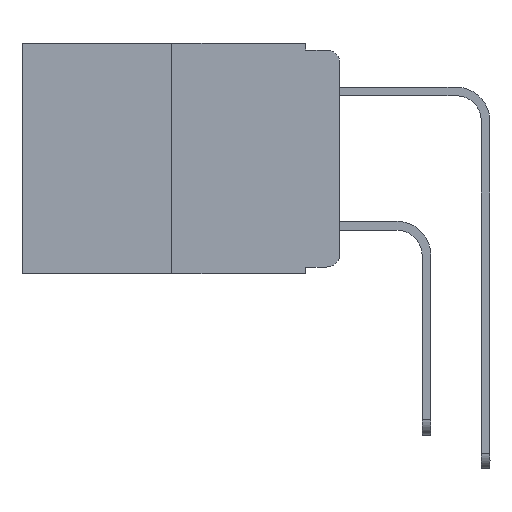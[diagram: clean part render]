
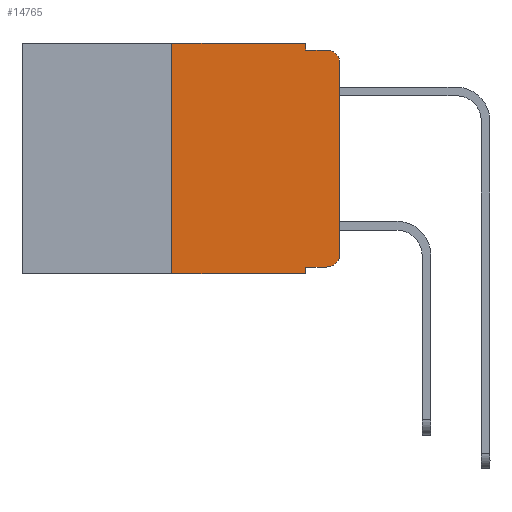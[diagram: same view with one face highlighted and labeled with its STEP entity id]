
A CAD part, left-side view. The second image highlights one B-rep face of the part: STEP entity #14765.
In plain terms, the highlighted planar face has unit normal (-1, 0, 0).
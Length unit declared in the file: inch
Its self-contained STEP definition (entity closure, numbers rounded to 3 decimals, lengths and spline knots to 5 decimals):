
#626 = EDGE_CURVE ( 'NONE', #15067, #20152, #23322, .T. ) ;
#967 = CARTESIAN_POINT ( 'NONE',  ( 0., 0.473, -0.343 ) ) ;
#976 = LINE ( 'NONE', #8235, #21357 ) ;
#1033 = CARTESIAN_POINT ( 'NONE',  ( 0., 0.25, 0. ) ) ;
#1343 = CARTESIAN_POINT ( 'NONE',  ( 0., 0.02, -0.01 ) ) ;
#1545 = VECTOR ( 'NONE', #8226, 39.37008 ) ;
#1653 = DIRECTION ( 'NONE',  ( 1., 0., 0. ) ) ;
#2267 = CARTESIAN_POINT ( 'NONE',  ( 0., 0.25, -0.343 ) ) ;
#2646 = EDGE_CURVE ( 'NONE', #20651, #21626, #9821, .T. ) ;
#3787 = LINE ( 'NONE', #14858, #6546 ) ;
#4066 = CARTESIAN_POINT ( 'NONE',  ( 0., 0.051, -0.343 ) ) ;
#4299 = DIRECTION ( 'NONE',  ( 0., 0., -1. ) ) ;
#4442 = ORIENTED_EDGE ( 'NONE', *, *, #7198, .T. ) ;
#4730 = ORIENTED_EDGE ( 'NONE', *, *, #15929, .F. ) ;
#5093 = FACE_OUTER_BOUND ( 'NONE', #17542, .T. ) ;
#5841 = VERTEX_POINT ( 'NONE', #2267 ) ;
#6095 = DIRECTION ( 'NONE',  ( -1., 0., 0. ) ) ;
#6388 = DIRECTION ( 'NONE',  ( 0., 0., -1. ) ) ;
#6546 = VECTOR ( 'NONE', #22117, 39.37008 ) ;
#6837 = CARTESIAN_POINT ( 'NONE',  ( 0., 0., 0. ) ) ;
#7178 = CARTESIAN_POINT ( 'NONE',  ( 0., 0., -0.313 ) ) ;
#7198 = EDGE_CURVE ( 'NONE', #5841, #21257, #10024, .T. ) ;
#7481 = EDGE_CURVE ( 'NONE', #10925, #21257, #3787, .T. ) ;
#7875 = DIRECTION ( 'NONE',  ( 0., -1., 0. ) ) ;
#8182 = EDGE_CURVE ( 'NONE', #10925, #9859, #14806, .T. ) ;
#8226 = DIRECTION ( 'NONE',  ( 0., -1., 0. ) ) ;
#8235 = CARTESIAN_POINT ( 'NONE',  ( 0., 0.051, -0.01 ) ) ;
#8594 = CARTESIAN_POINT ( 'NONE',  ( 0., 0.473, 0. ) ) ;
#9014 = CARTESIAN_POINT ( 'NONE',  ( 0., 0.25, 0. ) ) ;
#9821 = CIRCLE ( 'NONE', #10200, 0.02 ) ;
#9859 = VERTEX_POINT ( 'NONE', #19566 ) ;
#10024 = LINE ( 'NONE', #967, #1545 ) ;
#10200 = AXIS2_PLACEMENT_3D ( 'NONE', #11868, #22697, #6388 ) ;
#10466 = PLANE ( 'NONE',  #20581 ) ;
#10925 = VERTEX_POINT ( 'NONE', #15297 ) ;
#11100 = ORIENTED_EDGE ( 'NONE', *, *, #7481, .F. ) ;
#11280 = EDGE_CURVE ( 'NONE', #9859, #23039, #17438, .T. ) ;
#11868 = CARTESIAN_POINT ( 'NONE',  ( 0., 0.02, -0.03 ) ) ;
#11890 = VECTOR ( 'NONE', #17702, 39.37008 ) ;
#12331 = ORIENTED_EDGE ( 'NONE', *, *, #2646, .T. ) ;
#14676 = LINE ( 'NONE', #21932, #22485 ) ;
#14765 = ADVANCED_FACE ( 'NONE', ( #5093 ), #10466, .F. ) ;
#14806 = LINE ( 'NONE', #20512, #22334 ) ;
#14858 = CARTESIAN_POINT ( 'NONE',  ( 0., 0.051, 0. ) ) ;
#14924 = DIRECTION ( 'NONE',  ( 0., -1., 0. ) ) ;
#15067 = VERTEX_POINT ( 'NONE', #1033 ) ;
#15201 = ORIENTED_EDGE ( 'NONE', *, *, #16995, .F. ) ;
#15297 = CARTESIAN_POINT ( 'NONE',  ( 0., 0.051, -0.333 ) ) ;
#15801 = EDGE_CURVE ( 'NONE', #20152, #18317, #14676, .T. ) ;
#15929 = EDGE_CURVE ( 'NONE', #18317, #21626, #976, .T. ) ;
#16411 = CARTESIAN_POINT ( 'NONE',  ( 0., 0.473, 0. ) ) ;
#16995 = EDGE_CURVE ( 'NONE', #5841, #15067, #19829, .T. ) ;
#17438 = CIRCLE ( 'NONE', #22368, 0.02 ) ;
#17526 = CARTESIAN_POINT ( 'NONE',  ( 0., 0.02, -0.313 ) ) ;
#17542 = EDGE_LOOP ( 'NONE', ( #22169, #12331, #4730, #17608, #20171, #15201, #4442, #11100, #23228, #19562 ) ) ;
#17608 = ORIENTED_EDGE ( 'NONE', *, *, #15801, .F. ) ;
#17702 = DIRECTION ( 'NONE',  ( 0., 0., 1. ) ) ;
#18317 = VERTEX_POINT ( 'NONE', #22249 ) ;
#18590 = DIRECTION ( 'NONE',  ( 0., 0., -1. ) ) ;
#18980 = EDGE_CURVE ( 'NONE', #23039, #20651, #19689, .T. ) ;
#19372 = CARTESIAN_POINT ( 'NONE',  ( 0., 0.051, 0. ) ) ;
#19562 = ORIENTED_EDGE ( 'NONE', *, *, #11280, .T. ) ;
#19566 = CARTESIAN_POINT ( 'NONE',  ( 0., 0.02, -0.333 ) ) ;
#19625 = DIRECTION ( 'NONE',  ( 0., 0., -1. ) ) ;
#19689 = LINE ( 'NONE', #6837, #21075 ) ;
#19829 = LINE ( 'NONE', #9014, #11890 ) ;
#19994 = DIRECTION ( 'NONE',  ( 0., -1., 0. ) ) ;
#20152 = VERTEX_POINT ( 'NONE', #19372 ) ;
#20171 = ORIENTED_EDGE ( 'NONE', *, *, #626, .F. ) ;
#20512 = CARTESIAN_POINT ( 'NONE',  ( 0., 0.051, -0.333 ) ) ;
#20581 = AXIS2_PLACEMENT_3D ( 'NONE', #16411, #1653, #19625 ) ;
#20651 = VERTEX_POINT ( 'NONE', #22381 ) ;
#21075 = VECTOR ( 'NONE', #21240, 39.37008 ) ;
#21240 = DIRECTION ( 'NONE',  ( 0., 0., 1. ) ) ;
#21257 = VERTEX_POINT ( 'NONE', #4066 ) ;
#21357 = VECTOR ( 'NONE', #7875, 39.37008 ) ;
#21626 = VERTEX_POINT ( 'NONE', #1343 ) ;
#21932 = CARTESIAN_POINT ( 'NONE',  ( 0., 0.051, 0. ) ) ;
#22117 = DIRECTION ( 'NONE',  ( 0., 0., -1. ) ) ;
#22169 = ORIENTED_EDGE ( 'NONE', *, *, #18980, .T. ) ;
#22249 = CARTESIAN_POINT ( 'NONE',  ( 0., 0.051, -0.01 ) ) ;
#22334 = VECTOR ( 'NONE', #14924, 39.37008 ) ;
#22368 = AXIS2_PLACEMENT_3D ( 'NONE', #17526, #6095, #4299 ) ;
#22381 = CARTESIAN_POINT ( 'NONE',  ( 0., 0., -0.03 ) ) ;
#22485 = VECTOR ( 'NONE', #18590, 39.37008 ) ;
#22510 = VECTOR ( 'NONE', #19994, 39.37008 ) ;
#22697 = DIRECTION ( 'NONE',  ( -1., 0., 0. ) ) ;
#23039 = VERTEX_POINT ( 'NONE', #7178 ) ;
#23228 = ORIENTED_EDGE ( 'NONE', *, *, #8182, .T. ) ;
#23322 = LINE ( 'NONE', #8594, #22510 ) ;
